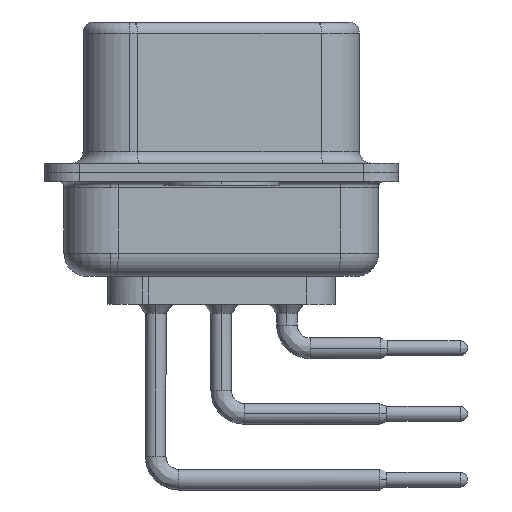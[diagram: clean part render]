
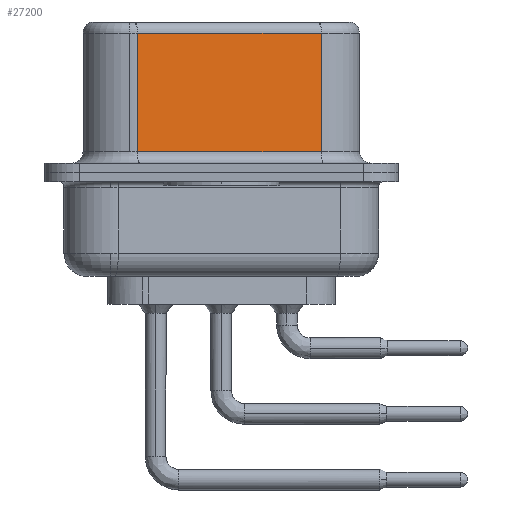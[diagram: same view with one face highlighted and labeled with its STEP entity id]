
A CAD part, left-side view. The second image highlights one B-rep face of the part: STEP entity #27200.
In plain terms, the highlighted planar face has unit normal (-0.985, -0.174, 0).
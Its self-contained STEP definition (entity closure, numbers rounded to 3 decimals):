
#1354 = DIRECTION ( 'NONE',  ( 0., 0., -1. ) ) ;
#2169 = EDGE_CURVE ( 'NONE', #15994, #11053, #23338, .T. ) ;
#4424 = VERTEX_POINT ( 'NONE', #14231 ) ;
#4757 = ORIENTED_EDGE ( 'NONE', *, *, #19044, .T. ) ;
#5387 = ORIENTED_EDGE ( 'NONE', *, *, #2169, .F. ) ;
#6761 = VECTOR ( 'NONE', #20860, 1000. ) ;
#6829 = CARTESIAN_POINT ( 'NONE',  ( 3.73, 3.628, 6.52 ) ) ;
#6965 = EDGE_LOOP ( 'NONE', ( #5387, #23662, #4757, #33757 ) ) ;
#7231 = CARTESIAN_POINT ( 'NONE',  ( 5.132, -4.322, 6.52 ) ) ;
#7352 = DIRECTION ( 'NONE',  ( -0.174, 0.985, 0. ) ) ;
#11053 = VERTEX_POINT ( 'NONE', #23240 ) ;
#12392 = CARTESIAN_POINT ( 'NONE',  ( 5.132, -4.322, 0.9 ) ) ;
#14097 = LINE ( 'NONE', #31491, #6761 ) ;
#14231 = CARTESIAN_POINT ( 'NONE',  ( 3.73, 3.628, 0.9 ) ) ;
#15994 = VERTEX_POINT ( 'NONE', #28981 ) ;
#16063 = VECTOR ( 'NONE', #29466, 1000. ) ;
#16207 = VERTEX_POINT ( 'NONE', #19344 ) ;
#17678 = VECTOR ( 'NONE', #28654, 1000. ) ;
#19044 = EDGE_CURVE ( 'NONE', #16207, #4424, #29931, .T. ) ;
#19344 = CARTESIAN_POINT ( 'NONE',  ( 3.73, 3.628, 6.02 ) ) ;
#20860 = DIRECTION ( 'NONE',  ( -0.174, 0.985, 0. ) ) ;
#21992 = VECTOR ( 'NONE', #1354, 1000. ) ;
#22781 = EDGE_CURVE ( 'NONE', #4424, #11053, #31121, .T. ) ;
#23157 = AXIS2_PLACEMENT_3D ( 'NONE', #7231, #23791, #7352 ) ;
#23240 = CARTESIAN_POINT ( 'NONE',  ( 5.132, -4.322, 0.9 ) ) ;
#23338 = LINE ( 'NONE', #29396, #16063 ) ;
#23662 = ORIENTED_EDGE ( 'NONE', *, *, #30528, .T. ) ;
#23791 = DIRECTION ( 'NONE',  ( 0.985, 0.174, 0. ) ) ;
#25877 = FACE_OUTER_BOUND ( 'NONE', #6965, .T. ) ;
#27200 = ADVANCED_FACE ( 'NONE', ( #25877 ), #31719, .F. ) ;
#28654 = DIRECTION ( 'NONE',  ( 0.174, -0.985, 0. ) ) ;
#28981 = CARTESIAN_POINT ( 'NONE',  ( 5.132, -4.322, 6.02 ) ) ;
#29396 = CARTESIAN_POINT ( 'NONE',  ( 5.132, -4.322, 6.52 ) ) ;
#29466 = DIRECTION ( 'NONE',  ( 0., 0., -1. ) ) ;
#29931 = LINE ( 'NONE', #6829, #21992 ) ;
#30528 = EDGE_CURVE ( 'NONE', #15994, #16207, #14097, .T. ) ;
#31121 = LINE ( 'NONE', #12392, #17678 ) ;
#31491 = CARTESIAN_POINT ( 'NONE',  ( 5.132, -4.322, 6.02 ) ) ;
#31719 = PLANE ( 'NONE',  #23157 ) ;
#33757 = ORIENTED_EDGE ( 'NONE', *, *, #22781, .T. ) ;
